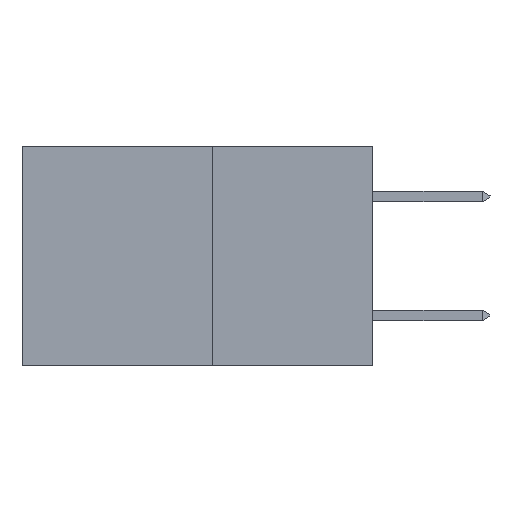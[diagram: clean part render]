
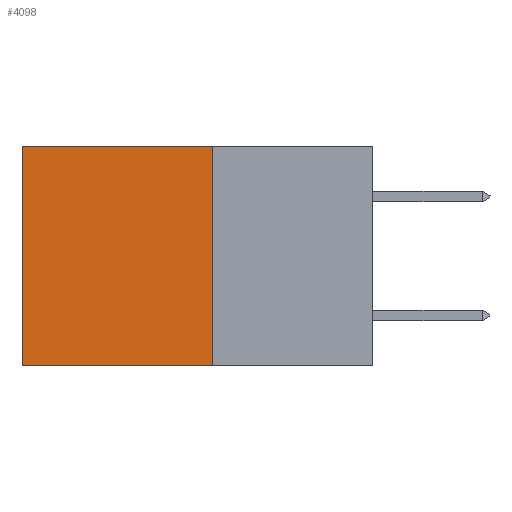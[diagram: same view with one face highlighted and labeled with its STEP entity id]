
A CAD part, left-side view. The second image highlights one B-rep face of the part: STEP entity #4098.
In plain terms, the highlighted planar face has unit normal (-1, 0, 0).
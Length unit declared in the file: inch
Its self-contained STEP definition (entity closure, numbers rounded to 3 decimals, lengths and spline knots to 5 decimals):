
#1325 = DIRECTION ( 'NONE',  ( 0., 0., -1. ) ) ;
#1938 = CARTESIAN_POINT ( 'NONE',  ( 0.277, 0.27, -0.37 ) ) ;
#2005 = CARTESIAN_POINT ( 'NONE',  ( 0.277, 0.27, -0.37 ) ) ;
#2494 = ORIENTED_EDGE ( 'NONE', *, *, #6116, .F. ) ;
#3119 = VECTOR ( 'NONE', #4818, 39.37008 ) ;
#3270 = CARTESIAN_POINT ( 'NONE',  ( 0.277, 0.27, 0. ) ) ;
#3513 = DIRECTION ( 'NONE',  ( 0., 0., -1. ) ) ;
#3683 = CARTESIAN_POINT ( 'NONE',  ( 0.277, 0.27, -0.37 ) ) ;
#4098 = ADVANCED_FACE ( 'NONE', ( #6074 ), #9351, .F. ) ;
#4130 = LINE ( 'NONE', #7932, #15509 ) ;
#4236 = EDGE_LOOP ( 'NONE', ( #10643, #6592, #2494, #17569 ) ) ;
#4817 = LINE ( 'NONE', #3683, #12019 ) ;
#4818 = DIRECTION ( 'NONE',  ( 0., 1., 0. ) ) ;
#5919 = VECTOR ( 'NONE', #1325, 39.37008 ) ;
#6074 = FACE_OUTER_BOUND ( 'NONE', #4236, .T. ) ;
#6116 = EDGE_CURVE ( 'NONE', #16202, #10150, #4130, .T. ) ;
#6592 = ORIENTED_EDGE ( 'NONE', *, *, #8003, .F. ) ;
#7552 = LINE ( 'NONE', #3270, #3119 ) ;
#7932 = CARTESIAN_POINT ( 'NONE',  ( 0.277, 0.27, -0.37 ) ) ;
#8003 = EDGE_CURVE ( 'NONE', #10150, #11071, #4817, .T. ) ;
#8879 = CARTESIAN_POINT ( 'NONE',  ( 0.277, 0.27, 0. ) ) ;
#8905 = EDGE_CURVE ( 'NONE', #13868, #11071, #17524, .T. ) ;
#9351 = PLANE ( 'NONE',  #17332 ) ;
#9569 = DIRECTION ( 'NONE',  ( 0., 1., 0. ) ) ;
#10150 = VERTEX_POINT ( 'NONE', #1938 ) ;
#10643 = ORIENTED_EDGE ( 'NONE', *, *, #8905, .T. ) ;
#11071 = VERTEX_POINT ( 'NONE', #16836 ) ;
#12019 = VECTOR ( 'NONE', #9569, 39.37008 ) ;
#12207 = DIRECTION ( 'NONE',  ( 1., 0., 0. ) ) ;
#12985 = CARTESIAN_POINT ( 'NONE',  ( 0.277, 0.59, -0.37 ) ) ;
#13868 = VERTEX_POINT ( 'NONE', #14452 ) ;
#14452 = CARTESIAN_POINT ( 'NONE',  ( 0.277, 0.59, 0. ) ) ;
#15509 = VECTOR ( 'NONE', #17616, 39.37008 ) ;
#16202 = VERTEX_POINT ( 'NONE', #8879 ) ;
#16836 = CARTESIAN_POINT ( 'NONE',  ( 0.277, 0.59, -0.37 ) ) ;
#17332 = AXIS2_PLACEMENT_3D ( 'NONE', #2005, #12207, #3513 ) ;
#17524 = LINE ( 'NONE', #12985, #5919 ) ;
#17569 = ORIENTED_EDGE ( 'NONE', *, *, #17793, .T. ) ;
#17616 = DIRECTION ( 'NONE',  ( 0., 0., -1. ) ) ;
#17793 = EDGE_CURVE ( 'NONE', #16202, #13868, #7552, .T. ) ;
